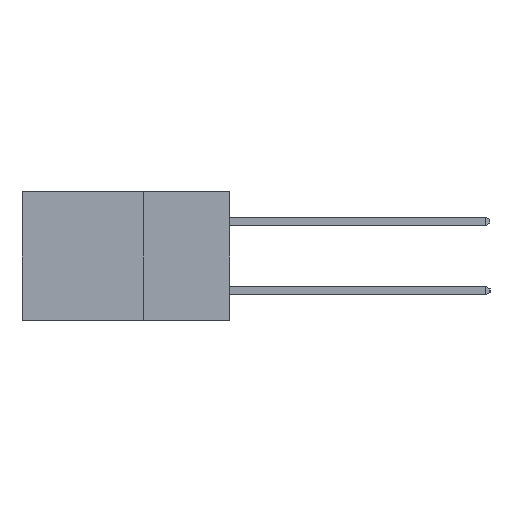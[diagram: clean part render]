
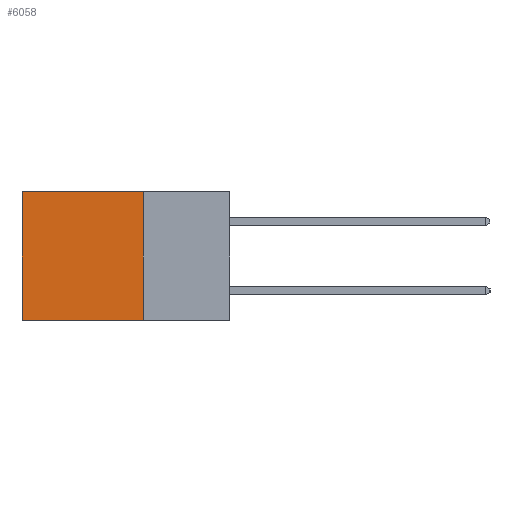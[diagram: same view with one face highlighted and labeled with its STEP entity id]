
A CAD part, left-side view. The second image highlights one B-rep face of the part: STEP entity #6058.
In plain terms, the highlighted planar face has unit normal (-1, 0, 0).
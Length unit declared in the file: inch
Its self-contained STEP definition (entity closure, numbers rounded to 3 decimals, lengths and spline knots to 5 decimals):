
#368 = ORIENTED_EDGE ( 'NONE', *, *, #8530, .T. ) ;
#570 = VECTOR ( 'NONE', #10583, 39.37008 ) ;
#621 = LINE ( 'NONE', #4965, #12093 ) ;
#787 = VERTEX_POINT ( 'NONE', #13567 ) ;
#914 = FACE_OUTER_BOUND ( 'NONE', #10743, .T. ) ;
#1019 = VERTEX_POINT ( 'NONE', #13142 ) ;
#1857 = EDGE_CURVE ( 'NONE', #1019, #2397, #10940, .T. ) ;
#2037 = LINE ( 'NONE', #10703, #570 ) ;
#2397 = VERTEX_POINT ( 'NONE', #9351 ) ;
#2455 = EDGE_CURVE ( 'NONE', #1019, #787, #621, .T. ) ;
#2457 = AXIS2_PLACEMENT_3D ( 'NONE', #13117, #13100, #13049 ) ;
#2641 = CARTESIAN_POINT ( 'NONE',  ( 0.2615, 0.25, -0.37 ) ) ;
#3039 = DIRECTION ( 'NONE',  ( 0., 0., -1. ) ) ;
#3203 = CARTESIAN_POINT ( 'NONE',  ( 0.2615, 0.6, -0.37 ) ) ;
#3975 = VECTOR ( 'NONE', #3039, 39.37008 ) ;
#4965 = CARTESIAN_POINT ( 'NONE',  ( 0.2615, 0.25, 0. ) ) ;
#6058 = ADVANCED_FACE ( 'NONE', ( #914 ), #13147, .F. ) ;
#6276 = DIRECTION ( 'NONE',  ( 0., 1., 0. ) ) ;
#7096 = DIRECTION ( 'NONE',  ( 0., 0., -1. ) ) ;
#7199 = LINE ( 'NONE', #3203, #3975 ) ;
#8530 = EDGE_CURVE ( 'NONE', #787, #9666, #7199, .T. ) ;
#8931 = ORIENTED_EDGE ( 'NONE', *, *, #1857, .F. ) ;
#9033 = ORIENTED_EDGE ( 'NONE', *, *, #2455, .T. ) ;
#9351 = CARTESIAN_POINT ( 'NONE',  ( 0.2615, 0.25, -0.37 ) ) ;
#9666 = VERTEX_POINT ( 'NONE', #12343 ) ;
#10583 = DIRECTION ( 'NONE',  ( 0., 1., 0. ) ) ;
#10606 = VECTOR ( 'NONE', #7096, 39.37008 ) ;
#10703 = CARTESIAN_POINT ( 'NONE',  ( 0.2615, 0.25, -0.37 ) ) ;
#10743 = EDGE_LOOP ( 'NONE', ( #368, #11980, #8931, #9033 ) ) ;
#10940 = LINE ( 'NONE', #2641, #10606 ) ;
#11525 = EDGE_CURVE ( 'NONE', #2397, #9666, #2037, .T. ) ;
#11980 = ORIENTED_EDGE ( 'NONE', *, *, #11525, .F. ) ;
#12093 = VECTOR ( 'NONE', #6276, 39.37008 ) ;
#12343 = CARTESIAN_POINT ( 'NONE',  ( 0.2615, 0.6, -0.37 ) ) ;
#13049 = DIRECTION ( 'NONE',  ( 0., 0., -1. ) ) ;
#13100 = DIRECTION ( 'NONE',  ( 1., 0., 0. ) ) ;
#13117 = CARTESIAN_POINT ( 'NONE',  ( 0.2615, 0.25, -0.37 ) ) ;
#13142 = CARTESIAN_POINT ( 'NONE',  ( 0.2615, 0.25, 0. ) ) ;
#13147 = PLANE ( 'NONE',  #2457 ) ;
#13567 = CARTESIAN_POINT ( 'NONE',  ( 0.2615, 0.6, 0. ) ) ;
